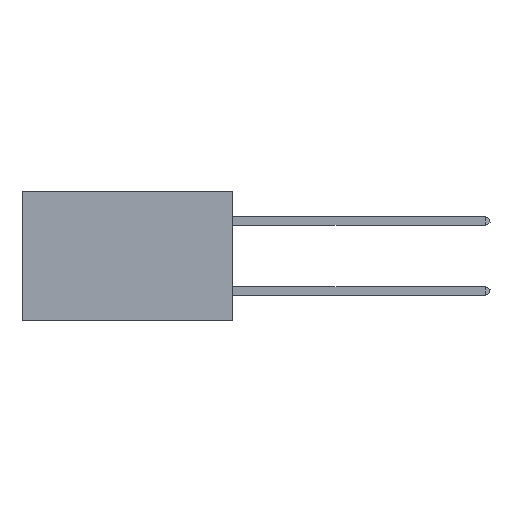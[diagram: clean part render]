
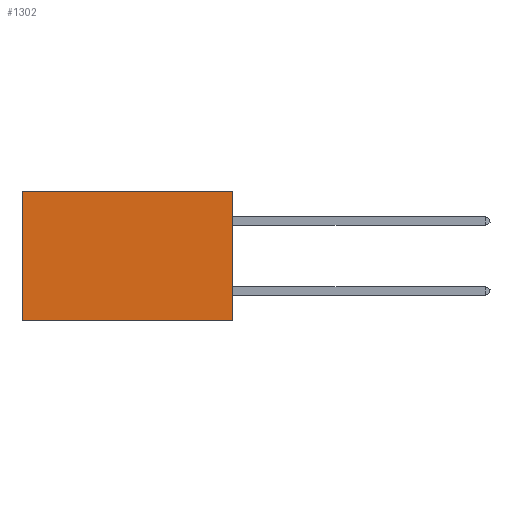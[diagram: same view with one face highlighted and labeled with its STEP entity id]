
A CAD part, left-side view. The second image highlights one B-rep face of the part: STEP entity #1302.
In plain terms, the highlighted planar face has unit normal (-1, 0, 0).
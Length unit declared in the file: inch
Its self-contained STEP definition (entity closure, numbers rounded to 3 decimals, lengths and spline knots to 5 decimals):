
#872 = CARTESIAN_POINT ( 'NONE',  ( 0.2875, 0., 0. ) ) ;
#919 = VECTOR ( 'NONE', #1247, 39.37008 ) ;
#1247 = DIRECTION ( 'NONE',  ( 0., 1., 0. ) ) ;
#1302 = ADVANCED_FACE ( 'NONE', ( #23706 ), #7079, .F. ) ;
#1800 = CARTESIAN_POINT ( 'NONE',  ( 0.2875, 0., -0.37 ) ) ;
#2261 = CARTESIAN_POINT ( 'NONE',  ( 0.2875, 0.6, 0. ) ) ;
#2795 = VERTEX_POINT ( 'NONE', #11169 ) ;
#3391 = AXIS2_PLACEMENT_3D ( 'NONE', #23723, #11351, #20696 ) ;
#4107 = ORIENTED_EDGE ( 'NONE', *, *, #23195, .T. ) ;
#4446 = VERTEX_POINT ( 'NONE', #1800 ) ;
#4596 = VECTOR ( 'NONE', #6311, 39.37008 ) ;
#5973 = EDGE_LOOP ( 'NONE', ( #19096, #18210, #19364, #4107 ) ) ;
#6311 = DIRECTION ( 'NONE',  ( 0., 0., -1. ) ) ;
#7079 = PLANE ( 'NONE',  #3391 ) ;
#7103 = CARTESIAN_POINT ( 'NONE',  ( 0.2875, 0., 0. ) ) ;
#8951 = VECTOR ( 'NONE', #14849, 39.37008 ) ;
#9205 = EDGE_CURVE ( 'NONE', #2795, #9358, #21746, .T. ) ;
#9358 = VERTEX_POINT ( 'NONE', #13844 ) ;
#9827 = EDGE_CURVE ( 'NONE', #4446, #9358, #13288, .T. ) ;
#11169 = CARTESIAN_POINT ( 'NONE',  ( 0.2875, 0.6, 0. ) ) ;
#11351 = DIRECTION ( 'NONE',  ( 1., 0., 0. ) ) ;
#11740 = LINE ( 'NONE', #17186, #22222 ) ;
#12930 = VERTEX_POINT ( 'NONE', #872 ) ;
#13288 = LINE ( 'NONE', #16799, #8951 ) ;
#13844 = CARTESIAN_POINT ( 'NONE',  ( 0.2875, 0.6, -0.37 ) ) ;
#13966 = LINE ( 'NONE', #7103, #919 ) ;
#14849 = DIRECTION ( 'NONE',  ( 0., 1., 0. ) ) ;
#16799 = CARTESIAN_POINT ( 'NONE',  ( 0.2875, 0., -0.37 ) ) ;
#17186 = CARTESIAN_POINT ( 'NONE',  ( 0.2875, 0., 0. ) ) ;
#18210 = ORIENTED_EDGE ( 'NONE', *, *, #9827, .F. ) ;
#19078 = DIRECTION ( 'NONE',  ( 0., 0., -1. ) ) ;
#19096 = ORIENTED_EDGE ( 'NONE', *, *, #9205, .T. ) ;
#19364 = ORIENTED_EDGE ( 'NONE', *, *, #19609, .F. ) ;
#19609 = EDGE_CURVE ( 'NONE', #12930, #4446, #11740, .T. ) ;
#20696 = DIRECTION ( 'NONE',  ( 0., 0., -1. ) ) ;
#21746 = LINE ( 'NONE', #2261, #4596 ) ;
#22222 = VECTOR ( 'NONE', #19078, 39.37008 ) ;
#23195 = EDGE_CURVE ( 'NONE', #12930, #2795, #13966, .T. ) ;
#23706 = FACE_OUTER_BOUND ( 'NONE', #5973, .T. ) ;
#23723 = CARTESIAN_POINT ( 'NONE',  ( 0.2875, 0., 0. ) ) ;
